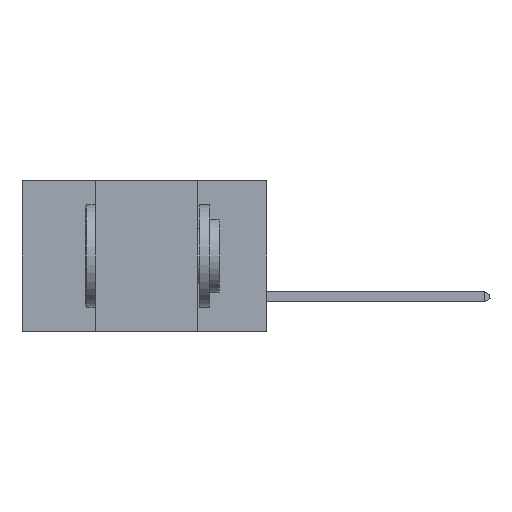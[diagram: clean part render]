
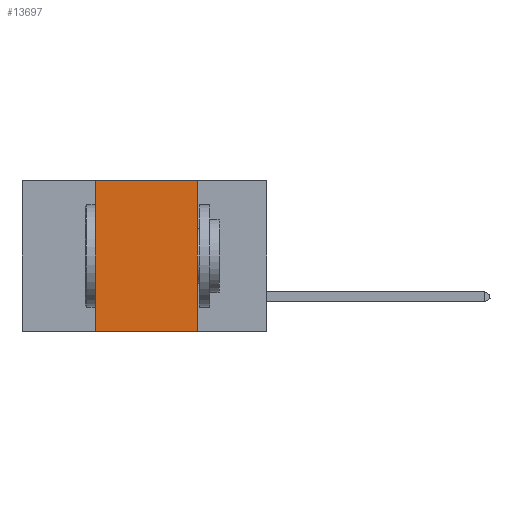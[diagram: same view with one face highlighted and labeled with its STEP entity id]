
A CAD part, left-side view. The second image highlights one B-rep face of the part: STEP entity #13697.
In plain terms, the highlighted planar face has unit normal (-1, 0, 0).
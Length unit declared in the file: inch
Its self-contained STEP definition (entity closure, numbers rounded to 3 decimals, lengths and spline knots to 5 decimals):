
#926 = CARTESIAN_POINT ( 'NONE',  ( 0., 0.42, 0. ) ) ;
#2128 = LINE ( 'NONE', #31154, #27898 ) ;
#2786 = VERTEX_POINT ( 'NONE', #26947 ) ;
#4372 = DIRECTION ( 'NONE',  ( 0., 0., 1. ) ) ;
#6473 = CARTESIAN_POINT ( 'NONE',  ( 0., 0.6, -0.37 ) ) ;
#7568 = PLANE ( 'NONE',  #13611 ) ;
#9959 = VECTOR ( 'NONE', #16426, 39.37008 ) ;
#10774 = DIRECTION ( 'NONE',  ( 1., 0., 0. ) ) ;
#11979 = EDGE_CURVE ( 'NONE', #35560, #2786, #31113, .T. ) ;
#11992 = VERTEX_POINT ( 'NONE', #926 ) ;
#13173 = CARTESIAN_POINT ( 'NONE',  ( 0., 0.6, 0. ) ) ;
#13611 = AXIS2_PLACEMENT_3D ( 'NONE', #31075, #10774, #14297 ) ;
#13697 = ADVANCED_FACE ( 'NONE', ( #24693 ), #7568, .F. ) ;
#13775 = CARTESIAN_POINT ( 'NONE',  ( 0., 0.17, 0. ) ) ;
#14297 = DIRECTION ( 'NONE',  ( 0., 0., -1. ) ) ;
#14780 = ORIENTED_EDGE ( 'NONE', *, *, #33636, .F. ) ;
#15466 = CARTESIAN_POINT ( 'NONE',  ( 0., 0.17, 0. ) ) ;
#16172 = ORIENTED_EDGE ( 'NONE', *, *, #29934, .T. ) ;
#16426 = DIRECTION ( 'NONE',  ( 0., -1., 0. ) ) ;
#24551 = VECTOR ( 'NONE', #41100, 39.37008 ) ;
#24693 = FACE_OUTER_BOUND ( 'NONE', #42272, .T. ) ;
#25656 = VERTEX_POINT ( 'NONE', #27379 ) ;
#26947 = CARTESIAN_POINT ( 'NONE',  ( 0., 0.17, -0.37 ) ) ;
#27379 = CARTESIAN_POINT ( 'NONE',  ( 0., 0.42, -0.37 ) ) ;
#27898 = VECTOR ( 'NONE', #4372, 39.37008 ) ;
#29934 = EDGE_CURVE ( 'NONE', #25656, #2786, #40288, .T. ) ;
#31075 = CARTESIAN_POINT ( 'NONE',  ( 0., 0.6, 0. ) ) ;
#31113 = LINE ( 'NONE', #15466, #38975 ) ;
#31154 = CARTESIAN_POINT ( 'NONE',  ( 0., 0.42, 0. ) ) ;
#33636 = EDGE_CURVE ( 'NONE', #25656, #11992, #2128, .T. ) ;
#34372 = EDGE_CURVE ( 'NONE', #11992, #35560, #36779, .T. ) ;
#35560 = VERTEX_POINT ( 'NONE', #13775 ) ;
#36779 = LINE ( 'NONE', #13173, #9959 ) ;
#37486 = ORIENTED_EDGE ( 'NONE', *, *, #11979, .F. ) ;
#37811 = DIRECTION ( 'NONE',  ( 0., 0., -1. ) ) ;
#38975 = VECTOR ( 'NONE', #37811, 39.37008 ) ;
#40288 = LINE ( 'NONE', #6473, #24551 ) ;
#41100 = DIRECTION ( 'NONE',  ( 0., -1., 0. ) ) ;
#42272 = EDGE_LOOP ( 'NONE', ( #37486, #43500, #14780, #16172 ) ) ;
#43500 = ORIENTED_EDGE ( 'NONE', *, *, #34372, .F. ) ;
